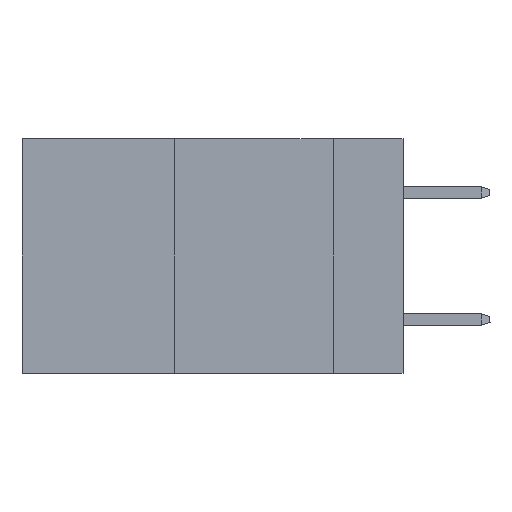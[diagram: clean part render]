
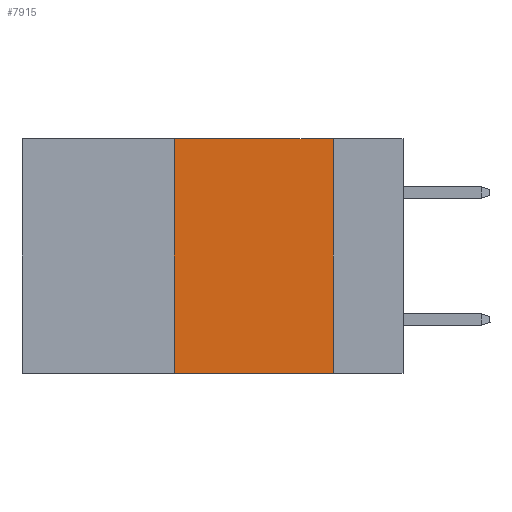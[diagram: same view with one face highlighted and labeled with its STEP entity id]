
A CAD part, left-side view. The second image highlights one B-rep face of the part: STEP entity #7915.
In plain terms, the highlighted planar face has unit normal (-1, 0, 0).
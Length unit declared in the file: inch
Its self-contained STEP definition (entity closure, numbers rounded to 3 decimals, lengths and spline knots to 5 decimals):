
#1136 = VECTOR ( 'NONE', #4760, 39.37008 ) ;
#1524 = CARTESIAN_POINT ( 'NONE',  ( 0., 0.11, -0.37 ) ) ;
#2804 = LINE ( 'NONE', #11538, #1136 ) ;
#2937 = DIRECTION ( 'NONE',  ( 0., 0., 1. ) ) ;
#3238 = ORIENTED_EDGE ( 'NONE', *, *, #9992, .F. ) ;
#4455 = CARTESIAN_POINT ( 'NONE',  ( 0., 0.6, 0. ) ) ;
#4760 = DIRECTION ( 'NONE',  ( 0., 0., -1. ) ) ;
#4866 = VECTOR ( 'NONE', #9850, 39.37008 ) ;
#6305 = PLANE ( 'NONE',  #9482 ) ;
#6423 = VERTEX_POINT ( 'NONE', #7617 ) ;
#6521 = LINE ( 'NONE', #12019, #4866 ) ;
#6882 = VERTEX_POINT ( 'NONE', #1524 ) ;
#7042 = EDGE_CURVE ( 'NONE', #13200, #6882, #6521, .T. ) ;
#7099 = EDGE_CURVE ( 'NONE', #6423, #11990, #11085, .T. ) ;
#7202 = CARTESIAN_POINT ( 'NONE',  ( 0., 0.11, 0. ) ) ;
#7617 = CARTESIAN_POINT ( 'NONE',  ( 0., 0.36, 0. ) ) ;
#7638 = ORIENTED_EDGE ( 'NONE', *, *, #7042, .T. ) ;
#7683 = DIRECTION ( 'NONE',  ( 1., 0., 0. ) ) ;
#7915 = ADVANCED_FACE ( 'NONE', ( #11820 ), #6305, .F. ) ;
#8172 = ORIENTED_EDGE ( 'NONE', *, *, #7099, .F. ) ;
#8907 = DIRECTION ( 'NONE',  ( 0., -1., 0. ) ) ;
#9043 = VECTOR ( 'NONE', #2937, 39.37008 ) ;
#9100 = EDGE_CURVE ( 'NONE', #13200, #6423, #10572, .T. ) ;
#9233 = VECTOR ( 'NONE', #8907, 39.37008 ) ;
#9249 = EDGE_LOOP ( 'NONE', ( #3238, #8172, #11035, #7638 ) ) ;
#9482 = AXIS2_PLACEMENT_3D ( 'NONE', #10722, #7683, #11947 ) ;
#9850 = DIRECTION ( 'NONE',  ( 0., -1., 0. ) ) ;
#9992 = EDGE_CURVE ( 'NONE', #11990, #6882, #2804, .T. ) ;
#10572 = LINE ( 'NONE', #11599, #9043 ) ;
#10722 = CARTESIAN_POINT ( 'NONE',  ( 0., 0.6, 0. ) ) ;
#11035 = ORIENTED_EDGE ( 'NONE', *, *, #9100, .F. ) ;
#11085 = LINE ( 'NONE', #4455, #9233 ) ;
#11538 = CARTESIAN_POINT ( 'NONE',  ( 0., 0.11, 0. ) ) ;
#11599 = CARTESIAN_POINT ( 'NONE',  ( 0., 0.36, 0. ) ) ;
#11820 = FACE_OUTER_BOUND ( 'NONE', #9249, .T. ) ;
#11908 = CARTESIAN_POINT ( 'NONE',  ( 0., 0.36, -0.37 ) ) ;
#11947 = DIRECTION ( 'NONE',  ( 0., 0., -1. ) ) ;
#11990 = VERTEX_POINT ( 'NONE', #7202 ) ;
#12019 = CARTESIAN_POINT ( 'NONE',  ( 0., 0.6, -0.37 ) ) ;
#13200 = VERTEX_POINT ( 'NONE', #11908 ) ;
